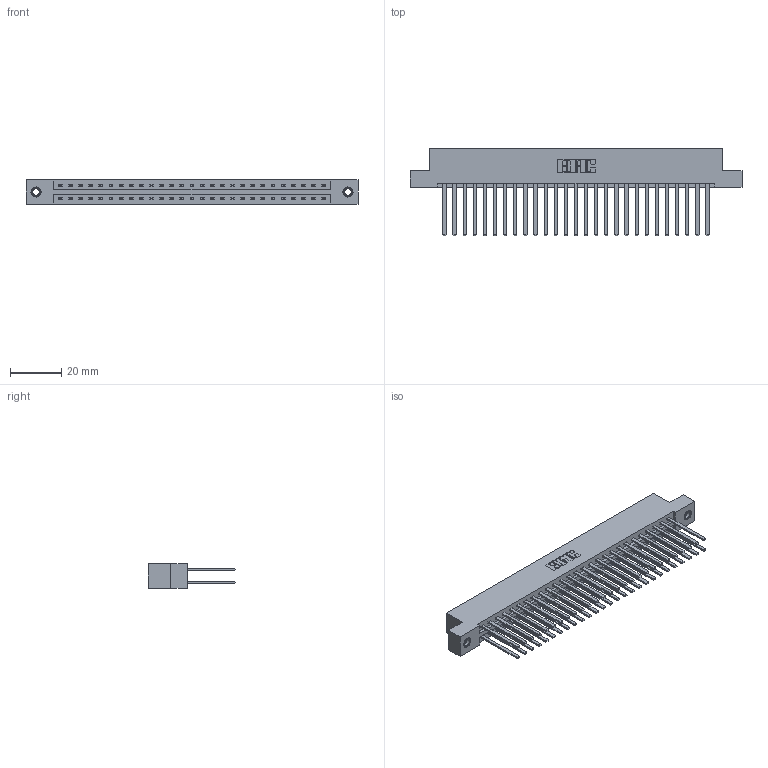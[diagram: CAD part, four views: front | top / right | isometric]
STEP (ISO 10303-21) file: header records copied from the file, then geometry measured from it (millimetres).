
FILE_DESCRIPTION (( 'STEP AP203' ), '1' );
FILE_NAME ('337-054-544-207.STEP', '2019-10-09T18:11:56', ( '' ), ( '' ), 'SwSTEP 2.0', 'SolidWorks 2016', '' );
FILE_SCHEMA (( 'CONFIG_CONTROL_DESIGN' ));
Length unit declared in the file: inch
Products named in the file (4): 337 Part_Flush Mounting Lugs - 0.156 Dia-TI; 337-054-544-207; 345-250-001_345-250-005-103; 345-292-001_345-293-144
Assembly tree (57 placements, depth 2):
  337-054-544-207
    337 Part_Flush Mounting Lugs - 0.156 Dia-TI
    345-292-001_345-293-144  x54
    345-250-001_345-250-005-103  x2
Bounding box: 130 x 34.3 x 9.4 mm (x, y, z)
Volume: 14243.9 mm3; surface area: 18465.9 mm2
Topology: 57 solids, 57 shells, 2766 faces, 8169 edges, 5366 vertices
Faces by surface type: plane 1938, cylinder 812, cone 12, torus 4
Entity records: 23876 total; most frequent: CARTESIAN_POINT 4013, ORIENTED_EDGE 3942, DIRECTION 3469, EDGE_CURVE 1971, VECTOR 1827, LINE 1827, VERTEX_POINT 1308, AXIS2_PLACEMENT_3D 821
